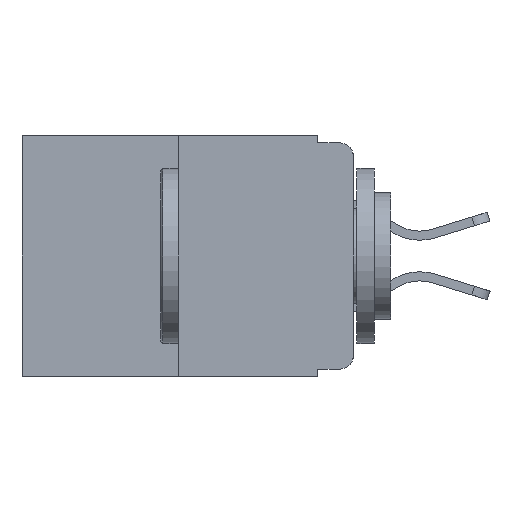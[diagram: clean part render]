
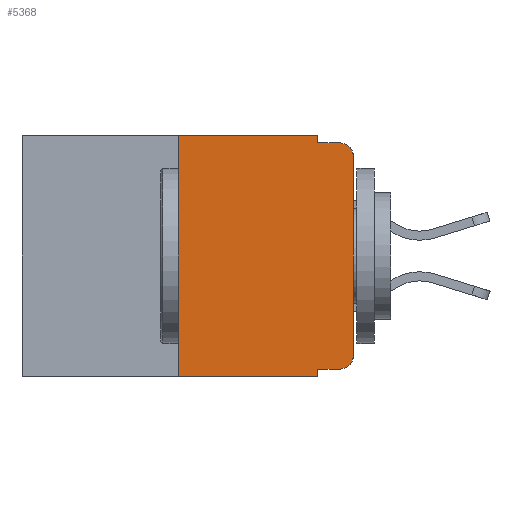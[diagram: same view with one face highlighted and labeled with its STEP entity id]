
A CAD part, left-side view. The second image highlights one B-rep face of the part: STEP entity #5368.
In plain terms, the highlighted planar face has unit normal (-1, 0, 0).
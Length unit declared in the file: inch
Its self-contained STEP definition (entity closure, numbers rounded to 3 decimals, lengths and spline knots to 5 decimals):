
#18 = CARTESIAN_POINT ( 'NONE',  ( 0., 0.051, -0.333 ) ) ;
#171 = VERTEX_POINT ( 'NONE', #7980 ) ;
#460 = LINE ( 'NONE', #7872, #11730 ) ;
#645 = CARTESIAN_POINT ( 'NONE',  ( 0., 0.25, 0. ) ) ;
#817 = LINE ( 'NONE', #9408, #14048 ) ;
#959 = DIRECTION ( 'NONE',  ( 0., 0., -1. ) ) ;
#1499 = VERTEX_POINT ( 'NONE', #12295 ) ;
#1776 = ORIENTED_EDGE ( 'NONE', *, *, #5965, .T. ) ;
#1790 = CARTESIAN_POINT ( 'NONE',  ( 0., 0.051, -0.01 ) ) ;
#1849 = CARTESIAN_POINT ( 'NONE',  ( 0., 0., -0.03 ) ) ;
#2137 = EDGE_CURVE ( 'NONE', #9294, #13267, #14686, .T. ) ;
#2422 = VERTEX_POINT ( 'NONE', #15842 ) ;
#2909 = ORIENTED_EDGE ( 'NONE', *, *, #8208, .T. ) ;
#3066 = CARTESIAN_POINT ( 'NONE',  ( 0., 0., -0.313 ) ) ;
#3260 = CARTESIAN_POINT ( 'NONE',  ( 0., 0.25, 0. ) ) ;
#3338 = LINE ( 'NONE', #18, #5536 ) ;
#3479 = EDGE_CURVE ( 'NONE', #14675, #2422, #10114, .T. ) ;
#4421 = VERTEX_POINT ( 'NONE', #11142 ) ;
#4692 = CARTESIAN_POINT ( 'NONE',  ( 0., 0.051, 0. ) ) ;
#5293 = AXIS2_PLACEMENT_3D ( 'NONE', #13582, #14696, #959 ) ;
#5344 = EDGE_CURVE ( 'NONE', #2422, #13267, #11149, .T. ) ;
#5368 = ADVANCED_FACE ( 'NONE', ( #6598 ), #5971, .F. ) ;
#5536 = VECTOR ( 'NONE', #12579, 39.37008 ) ;
#5575 = VECTOR ( 'NONE', #14826, 39.37008 ) ;
#5635 = DIRECTION ( 'NONE',  ( 0., -1., 0. ) ) ;
#5699 = VERTEX_POINT ( 'NONE', #3066 ) ;
#5965 = EDGE_CURVE ( 'NONE', #16000, #5699, #14285, .T. ) ;
#5971 = PLANE ( 'NONE',  #15680 ) ;
#6093 = ORIENTED_EDGE ( 'NONE', *, *, #7128, .T. ) ;
#6176 = DIRECTION ( 'NONE',  ( 0., 0., -1. ) ) ;
#6230 = ORIENTED_EDGE ( 'NONE', *, *, #5344, .F. ) ;
#6539 = DIRECTION ( 'NONE',  ( 0., -1., 0. ) ) ;
#6598 = FACE_OUTER_BOUND ( 'NONE', #11606, .T. ) ;
#6951 = EDGE_CURVE ( 'NONE', #171, #4421, #460, .T. ) ;
#7020 = EDGE_CURVE ( 'NONE', #171, #13434, #13662, .T. ) ;
#7128 = EDGE_CURVE ( 'NONE', #5699, #9294, #817, .T. ) ;
#7278 = CARTESIAN_POINT ( 'NONE',  ( 0., 0.473, 0. ) ) ;
#7319 = DIRECTION ( 'NONE',  ( -1., 0., 0. ) ) ;
#7872 = CARTESIAN_POINT ( 'NONE',  ( 0., 0.473, -0.343 ) ) ;
#7980 = CARTESIAN_POINT ( 'NONE',  ( 0., 0.25, -0.343 ) ) ;
#8035 = CARTESIAN_POINT ( 'NONE',  ( 0., 0.02, -0.01 ) ) ;
#8208 = EDGE_CURVE ( 'NONE', #1499, #16000, #3338, .T. ) ;
#8499 = CARTESIAN_POINT ( 'NONE',  ( 0., 0.051, 0. ) ) ;
#8834 = LINE ( 'NONE', #8499, #15361 ) ;
#8865 = EDGE_CURVE ( 'NONE', #13434, #14675, #15583, .T. ) ;
#8890 = DIRECTION ( 'NONE',  ( 0., -1., 0. ) ) ;
#9294 = VERTEX_POINT ( 'NONE', #1849 ) ;
#9408 = CARTESIAN_POINT ( 'NONE',  ( 0., 0., 0. ) ) ;
#9443 = ORIENTED_EDGE ( 'NONE', *, *, #3479, .F. ) ;
#9514 = DIRECTION ( 'NONE',  ( 0., 0., 1. ) ) ;
#9835 = EDGE_CURVE ( 'NONE', #1499, #4421, #8834, .T. ) ;
#9877 = AXIS2_PLACEMENT_3D ( 'NONE', #12444, #7319, #6176 ) ;
#10114 = LINE ( 'NONE', #11026, #5575 ) ;
#10215 = CARTESIAN_POINT ( 'NONE',  ( 0., 0.473, 0. ) ) ;
#10278 = ORIENTED_EDGE ( 'NONE', *, *, #9835, .F. ) ;
#10333 = VECTOR ( 'NONE', #14528, 39.37008 ) ;
#11026 = CARTESIAN_POINT ( 'NONE',  ( 0., 0.051, 0. ) ) ;
#11142 = CARTESIAN_POINT ( 'NONE',  ( 0., 0.051, -0.343 ) ) ;
#11149 = LINE ( 'NONE', #1790, #13687 ) ;
#11239 = VECTOR ( 'NONE', #8890, 39.37008 ) ;
#11271 = DIRECTION ( 'NONE',  ( 0., 0., -1. ) ) ;
#11606 = EDGE_LOOP ( 'NONE', ( #6093, #11680, #6230, #9443, #12631, #15069, #14439, #10278, #2909, #1776 ) ) ;
#11680 = ORIENTED_EDGE ( 'NONE', *, *, #2137, .T. ) ;
#11730 = VECTOR ( 'NONE', #6539, 39.37008 ) ;
#12252 = DIRECTION ( 'NONE',  ( 1., 0., 0. ) ) ;
#12295 = CARTESIAN_POINT ( 'NONE',  ( 0., 0.051, -0.333 ) ) ;
#12444 = CARTESIAN_POINT ( 'NONE',  ( 0., 0.02, -0.313 ) ) ;
#12579 = DIRECTION ( 'NONE',  ( 0., -1., 0. ) ) ;
#12631 = ORIENTED_EDGE ( 'NONE', *, *, #8865, .F. ) ;
#13267 = VERTEX_POINT ( 'NONE', #8035 ) ;
#13434 = VERTEX_POINT ( 'NONE', #3260 ) ;
#13582 = CARTESIAN_POINT ( 'NONE',  ( 0., 0.02, -0.03 ) ) ;
#13662 = LINE ( 'NONE', #645, #10333 ) ;
#13687 = VECTOR ( 'NONE', #5635, 39.37008 ) ;
#14048 = VECTOR ( 'NONE', #9514, 39.37008 ) ;
#14285 = CIRCLE ( 'NONE', #9877, 0.02 ) ;
#14439 = ORIENTED_EDGE ( 'NONE', *, *, #6951, .T. ) ;
#14528 = DIRECTION ( 'NONE',  ( 0., 0., 1. ) ) ;
#14675 = VERTEX_POINT ( 'NONE', #4692 ) ;
#14686 = CIRCLE ( 'NONE', #5293, 0.02 ) ;
#14696 = DIRECTION ( 'NONE',  ( -1., 0., 0. ) ) ;
#14799 = DIRECTION ( 'NONE',  ( 0., 0., -1. ) ) ;
#14826 = DIRECTION ( 'NONE',  ( 0., 0., -1. ) ) ;
#15069 = ORIENTED_EDGE ( 'NONE', *, *, #7020, .F. ) ;
#15361 = VECTOR ( 'NONE', #11271, 39.37008 ) ;
#15458 = CARTESIAN_POINT ( 'NONE',  ( 0., 0.02, -0.333 ) ) ;
#15583 = LINE ( 'NONE', #10215, #11239 ) ;
#15680 = AXIS2_PLACEMENT_3D ( 'NONE', #7278, #12252, #14799 ) ;
#15842 = CARTESIAN_POINT ( 'NONE',  ( 0., 0.051, -0.01 ) ) ;
#16000 = VERTEX_POINT ( 'NONE', #15458 ) ;
